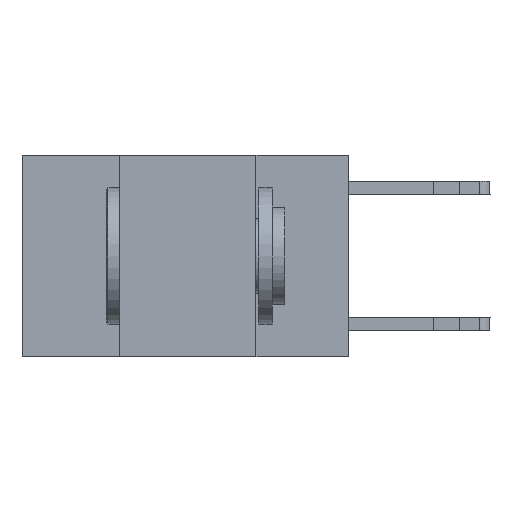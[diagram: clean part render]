
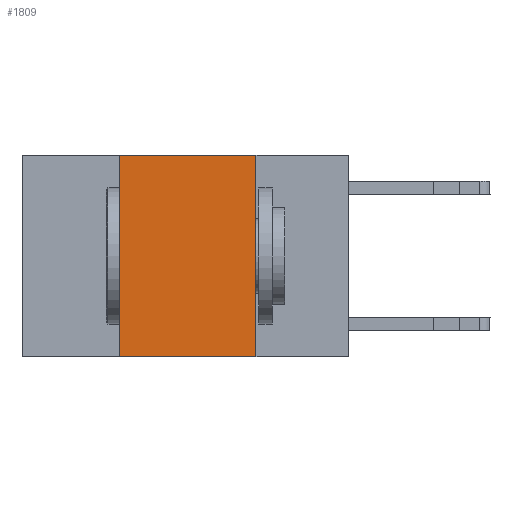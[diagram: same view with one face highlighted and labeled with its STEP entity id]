
A CAD part, left-side view. The second image highlights one B-rep face of the part: STEP entity #1809.
In plain terms, the highlighted planar face has unit normal (-1, 0, 0).
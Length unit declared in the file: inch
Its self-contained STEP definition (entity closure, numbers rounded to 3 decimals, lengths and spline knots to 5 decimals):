
#195 = EDGE_CURVE ( 'NONE', #3412, #16411, #11196, .T. ) ;
#1692 = LINE ( 'NONE', #3355, #11335 ) ;
#1809 = ADVANCED_FACE ( 'NONE', ( #6036 ), #7367, .F. ) ;
#2081 = EDGE_CURVE ( 'NONE', #14593, #14125, #1692, .T. ) ;
#2448 = DIRECTION ( 'NONE',  ( 0., 0., 1. ) ) ;
#3355 = CARTESIAN_POINT ( 'NONE',  ( 0., 0.17, 0. ) ) ;
#3412 = VERTEX_POINT ( 'NONE', #7443 ) ;
#4170 = VECTOR ( 'NONE', #2448, 39.37008 ) ;
#4273 = ORIENTED_EDGE ( 'NONE', *, *, #8460, .F. ) ;
#4523 = EDGE_LOOP ( 'NONE', ( #9735, #4273, #7711, #11190 ) ) ;
#4754 = DIRECTION ( 'NONE',  ( 0., 0., -1. ) ) ;
#6036 = FACE_OUTER_BOUND ( 'NONE', #4523, .T. ) ;
#6797 = DIRECTION ( 'NONE',  ( 0., 0., -1. ) ) ;
#7367 = PLANE ( 'NONE',  #15102 ) ;
#7443 = CARTESIAN_POINT ( 'NONE',  ( 0., 0.42, -0.37 ) ) ;
#7711 = ORIENTED_EDGE ( 'NONE', *, *, #195, .F. ) ;
#8185 = VECTOR ( 'NONE', #8681, 39.37008 ) ;
#8187 = LINE ( 'NONE', #12408, #13586 ) ;
#8460 = EDGE_CURVE ( 'NONE', #16411, #14593, #8187, .T. ) ;
#8633 = CARTESIAN_POINT ( 'NONE',  ( 0., 0.6, 0. ) ) ;
#8681 = DIRECTION ( 'NONE',  ( 0., -1., 0. ) ) ;
#8766 = LINE ( 'NONE', #9931, #8185 ) ;
#9071 = EDGE_CURVE ( 'NONE', #3412, #14125, #8766, .T. ) ;
#9735 = ORIENTED_EDGE ( 'NONE', *, *, #2081, .F. ) ;
#9931 = CARTESIAN_POINT ( 'NONE',  ( 0., 0.6, -0.37 ) ) ;
#11190 = ORIENTED_EDGE ( 'NONE', *, *, #9071, .T. ) ;
#11196 = LINE ( 'NONE', #11364, #4170 ) ;
#11335 = VECTOR ( 'NONE', #6797, 39.37008 ) ;
#11364 = CARTESIAN_POINT ( 'NONE',  ( 0., 0.42, 0. ) ) ;
#12408 = CARTESIAN_POINT ( 'NONE',  ( 0., 0.6, 0. ) ) ;
#13110 = CARTESIAN_POINT ( 'NONE',  ( 0., 0.17, 0. ) ) ;
#13586 = VECTOR ( 'NONE', #15025, 39.37008 ) ;
#14035 = DIRECTION ( 'NONE',  ( 1., 0., 0. ) ) ;
#14125 = VERTEX_POINT ( 'NONE', #15816 ) ;
#14593 = VERTEX_POINT ( 'NONE', #13110 ) ;
#15025 = DIRECTION ( 'NONE',  ( 0., -1., 0. ) ) ;
#15102 = AXIS2_PLACEMENT_3D ( 'NONE', #8633, #14035, #4754 ) ;
#15816 = CARTESIAN_POINT ( 'NONE',  ( 0., 0.17, -0.37 ) ) ;
#16411 = VERTEX_POINT ( 'NONE', #16549 ) ;
#16549 = CARTESIAN_POINT ( 'NONE',  ( 0., 0.42, 0. ) ) ;
